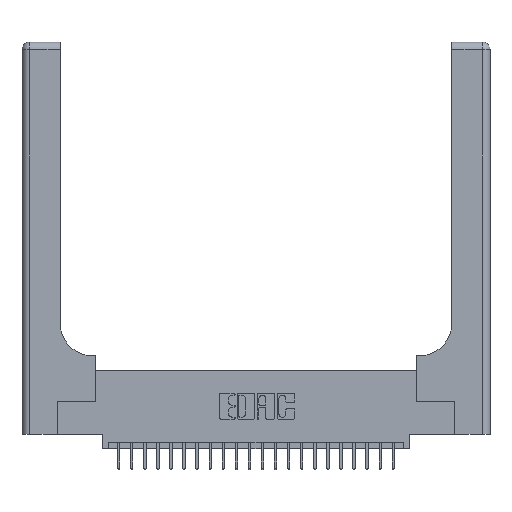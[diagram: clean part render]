
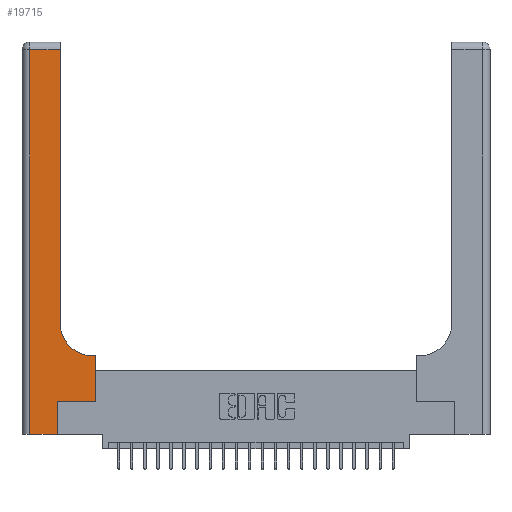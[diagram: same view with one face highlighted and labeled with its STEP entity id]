
A CAD part, top view. The second image highlights one B-rep face of the part: STEP entity #19715.
In plain terms, the highlighted planar face has unit normal (0, 0, 1).
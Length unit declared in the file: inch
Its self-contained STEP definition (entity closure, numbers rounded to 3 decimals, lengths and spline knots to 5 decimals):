
#426 = DIRECTION ( 'NONE',  ( 0., -1., 0. ) ) ;
#670 = DIRECTION ( 'NONE',  ( 0., 1., 0. ) ) ;
#742 = VERTEX_POINT ( 'NONE', #5455 ) ;
#1438 = ORIENTED_EDGE ( 'NONE', *, *, #12270, .T. ) ;
#2394 = PLANE ( 'NONE',  #22934 ) ;
#2562 = CARTESIAN_POINT ( 'NONE',  ( 0.06, 2.94, 0.37 ) ) ;
#2650 = LINE ( 'NONE', #16788, #11860 ) ;
#2810 = DIRECTION ( 'NONE',  ( -1., 0., 0. ) ) ;
#2976 = DIRECTION ( 'NONE',  ( 0., 0., -1. ) ) ;
#3832 = DIRECTION ( 'NONE',  ( 0., 1., 0. ) ) ;
#3898 = EDGE_CURVE ( 'NONE', #742, #9506, #9839, .T. ) ;
#5455 = CARTESIAN_POINT ( 'NONE',  ( 0.5415, 0.6, 0.37 ) ) ;
#5460 = LINE ( 'NONE', #18250, #15260 ) ;
#5551 = CARTESIAN_POINT ( 'NONE',  ( 0.269, 0.25, 0.37 ) ) ;
#5553 = VECTOR ( 'NONE', #8095, 39.37008 ) ;
#5723 = VECTOR ( 'NONE', #426, 39.37008 ) ;
#5971 = CARTESIAN_POINT ( 'NONE',  ( 0.5585, 0.25, 0.37 ) ) ;
#6027 = EDGE_CURVE ( 'NONE', #6334, #23635, #5460, .T. ) ;
#6165 = AXIS2_PLACEMENT_3D ( 'NONE', #13067, #10938, #8902 ) ;
#6334 = VERTEX_POINT ( 'NONE', #24957 ) ;
#6608 = EDGE_CURVE ( 'NONE', #17908, #11930, #23477, .T. ) ;
#7637 = EDGE_CURVE ( 'NONE', #12969, #12901, #2650, .T. ) ;
#7806 = CARTESIAN_POINT ( 'NONE',  ( 0.269, 0., 0.37 ) ) ;
#8002 = EDGE_LOOP ( 'NONE', ( #14468, #23185, #14252, #19290, #1438, #22065, #8835, #18111, #20471 ) ) ;
#8095 = DIRECTION ( 'NONE',  ( -1., 0., 0. ) ) ;
#8159 = DIRECTION ( 'NONE',  ( 1., 0., 0. ) ) ;
#8338 = CARTESIAN_POINT ( 'NONE',  ( 0.5585, 0.6, 0.37 ) ) ;
#8451 = VECTOR ( 'NONE', #11114, 39.37008 ) ;
#8835 = ORIENTED_EDGE ( 'NONE', *, *, #7637, .T. ) ;
#8902 = DIRECTION ( 'NONE',  ( 1., 0., 0. ) ) ;
#8969 = EDGE_CURVE ( 'NONE', #11930, #6334, #14913, .T. ) ;
#9506 = VERTEX_POINT ( 'NONE', #10083 ) ;
#9839 = CIRCLE ( 'NONE', #6165, 0.25 ) ;
#10083 = CARTESIAN_POINT ( 'NONE',  ( 0.2915, 0.85, 0.37 ) ) ;
#10117 = EDGE_CURVE ( 'NONE', #20540, #12969, #23105, .T. ) ;
#10232 = CARTESIAN_POINT ( 'NONE',  ( 0.2915, 0.6, 0.37 ) ) ;
#10289 = CARTESIAN_POINT ( 'NONE',  ( 0.2915, 3., 0.37 ) ) ;
#10938 = DIRECTION ( 'NONE',  ( 0., 0., -1. ) ) ;
#11114 = DIRECTION ( 'NONE',  ( 1., 0., 0. ) ) ;
#11860 = VECTOR ( 'NONE', #18681, 39.37008 ) ;
#11930 = VERTEX_POINT ( 'NONE', #2562 ) ;
#12270 = EDGE_CURVE ( 'NONE', #23635, #20540, #22170, .T. ) ;
#12793 = DIRECTION ( 'NONE',  ( -1., 0., 0. ) ) ;
#12901 = VERTEX_POINT ( 'NONE', #8338 ) ;
#12969 = VERTEX_POINT ( 'NONE', #5971 ) ;
#13067 = CARTESIAN_POINT ( 'NONE',  ( 0.5415, 0.85, 0.37 ) ) ;
#14252 = ORIENTED_EDGE ( 'NONE', *, *, #8969, .T. ) ;
#14468 = ORIENTED_EDGE ( 'NONE', *, *, #15047, .T. ) ;
#14515 = CARTESIAN_POINT ( 'NONE',  ( 0.269, 0., 0.37 ) ) ;
#14575 = FACE_OUTER_BOUND ( 'NONE', #8002, .T. ) ;
#14829 = VECTOR ( 'NONE', #3832, 39.37008 ) ;
#14913 = LINE ( 'NONE', #18074, #5723 ) ;
#15047 = EDGE_CURVE ( 'NONE', #9506, #17908, #22979, .T. ) ;
#15260 = VECTOR ( 'NONE', #8159, 39.37008 ) ;
#15682 = LINE ( 'NONE', #10232, #5553 ) ;
#16564 = VECTOR ( 'NONE', #670, 39.37008 ) ;
#16768 = VECTOR ( 'NONE', #12793, 39.37008 ) ;
#16788 = CARTESIAN_POINT ( 'NONE',  ( 0.5585, 0.25, 0.37 ) ) ;
#17908 = VERTEX_POINT ( 'NONE', #25015 ) ;
#17933 = CARTESIAN_POINT ( 'NONE',  ( 0., 3., 0.37 ) ) ;
#18074 = CARTESIAN_POINT ( 'NONE',  ( 0.06, 3., 0.37 ) ) ;
#18111 = ORIENTED_EDGE ( 'NONE', *, *, #22125, .T. ) ;
#18250 = CARTESIAN_POINT ( 'NONE',  ( 0., 0., 0.37 ) ) ;
#18681 = DIRECTION ( 'NONE',  ( 0., 1., 0. ) ) ;
#19290 = ORIENTED_EDGE ( 'NONE', *, *, #6027, .T. ) ;
#19715 = ADVANCED_FACE ( 'NONE', ( #14575 ), #2394, .F. ) ;
#20471 = ORIENTED_EDGE ( 'NONE', *, *, #3898, .T. ) ;
#20540 = VERTEX_POINT ( 'NONE', #22486 ) ;
#22065 = ORIENTED_EDGE ( 'NONE', *, *, #10117, .T. ) ;
#22125 = EDGE_CURVE ( 'NONE', #12901, #742, #15682, .T. ) ;
#22170 = LINE ( 'NONE', #7806, #14829 ) ;
#22472 = CARTESIAN_POINT ( 'NONE',  ( 0., 2.94, 0.37 ) ) ;
#22486 = CARTESIAN_POINT ( 'NONE',  ( 0.269, 0.25, 0.37 ) ) ;
#22934 = AXIS2_PLACEMENT_3D ( 'NONE', #17933, #2976, #2810 ) ;
#22979 = LINE ( 'NONE', #10289, #16564 ) ;
#23105 = LINE ( 'NONE', #5551, #8451 ) ;
#23185 = ORIENTED_EDGE ( 'NONE', *, *, #6608, .T. ) ;
#23477 = LINE ( 'NONE', #22472, #16768 ) ;
#23635 = VERTEX_POINT ( 'NONE', #14515 ) ;
#24957 = CARTESIAN_POINT ( 'NONE',  ( 0.06, 0., 0.37 ) ) ;
#25015 = CARTESIAN_POINT ( 'NONE',  ( 0.2915, 2.94, 0.37 ) ) ;
